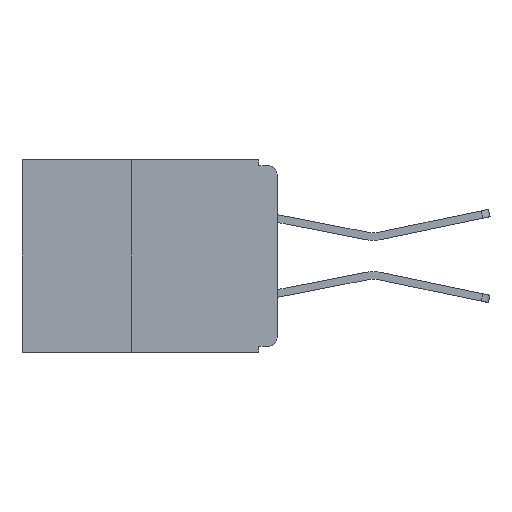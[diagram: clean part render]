
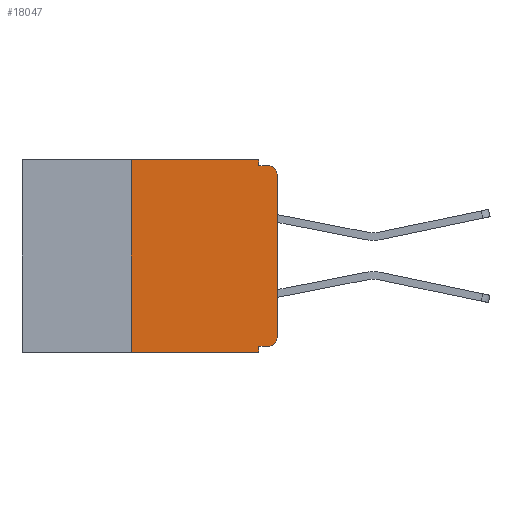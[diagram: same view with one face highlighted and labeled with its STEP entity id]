
A CAD part, left-side view. The second image highlights one B-rep face of the part: STEP entity #18047.
In plain terms, the highlighted planar face has unit normal (-1, 0, 0).
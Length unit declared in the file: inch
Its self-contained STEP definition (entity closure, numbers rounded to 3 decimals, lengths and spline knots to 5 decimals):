
#523 = VECTOR ( 'NONE', #11589, 39.37008 ) ;
#1470 = VERTEX_POINT ( 'NONE', #19646 ) ;
#1898 = VECTOR ( 'NONE', #27542, 39.37008 ) ;
#2054 = VECTOR ( 'NONE', #28961, 39.37008 ) ;
#2143 = VECTOR ( 'NONE', #12519, 39.37008 ) ;
#2217 = CIRCLE ( 'NONE', #30447, 0.015 ) ;
#2583 = ORIENTED_EDGE ( 'NONE', *, *, #22850, .F. ) ;
#2892 = VERTEX_POINT ( 'NONE', #30218 ) ;
#3573 = EDGE_CURVE ( 'NONE', #6749, #24442, #2217, .T. ) ;
#4048 = CARTESIAN_POINT ( 'NONE',  ( 0., 0.015, -0.01 ) ) ;
#4120 = DIRECTION ( 'NONE',  ( 0., 0., 1. ) ) ;
#5035 = VECTOR ( 'NONE', #14253, 39.37008 ) ;
#5167 = DIRECTION ( 'NONE',  ( 0., 0., -1. ) ) ;
#5255 = DIRECTION ( 'NONE',  ( -1., 0., 0. ) ) ;
#6128 = EDGE_CURVE ( 'NONE', #2892, #11223, #21045, .T. ) ;
#6496 = LINE ( 'NONE', #28523, #13029 ) ;
#6749 = VERTEX_POINT ( 'NONE', #17770 ) ;
#6940 = CARTESIAN_POINT ( 'NONE',  ( 0., 0.437, 0. ) ) ;
#6986 = CARTESIAN_POINT ( 'NONE',  ( 0., 0., -0.01 ) ) ;
#7570 = CARTESIAN_POINT ( 'NONE',  ( 0., 0.015, -0.32 ) ) ;
#8571 = LINE ( 'NONE', #6940, #2054 ) ;
#9008 = VERTEX_POINT ( 'NONE', #7570 ) ;
#9143 = CARTESIAN_POINT ( 'NONE',  ( 0., 0., -0.32 ) ) ;
#9176 = PLANE ( 'NONE',  #24827 ) ;
#9881 = CARTESIAN_POINT ( 'NONE',  ( 0., 0., -0.305 ) ) ;
#10434 = CARTESIAN_POINT ( 'NONE',  ( 0., 0.437, -0.33 ) ) ;
#10629 = CARTESIAN_POINT ( 'NONE',  ( 0., 0.25, -0.33 ) ) ;
#11039 = EDGE_CURVE ( 'NONE', #13516, #6749, #6496, .T. ) ;
#11223 = VERTEX_POINT ( 'NONE', #12266 ) ;
#11443 = VERTEX_POINT ( 'NONE', #30097 ) ;
#11589 = DIRECTION ( 'NONE',  ( 0., 1., 0. ) ) ;
#12009 = EDGE_CURVE ( 'NONE', #31217, #30993, #29386, .T. ) ;
#12266 = CARTESIAN_POINT ( 'NONE',  ( 0., 0.031, -0.33 ) ) ;
#12460 = CARTESIAN_POINT ( 'NONE',  ( 0., 0.031, -0.33 ) ) ;
#12519 = DIRECTION ( 'NONE',  ( 0., 0., -1. ) ) ;
#12658 = DIRECTION ( 'NONE',  ( 0., 0., 1. ) ) ;
#13029 = VECTOR ( 'NONE', #4120, 39.37008 ) ;
#13365 = LINE ( 'NONE', #10434, #1898 ) ;
#13516 = VERTEX_POINT ( 'NONE', #9881 ) ;
#14086 = CARTESIAN_POINT ( 'NONE',  ( 0., 0.437, 0. ) ) ;
#14253 = DIRECTION ( 'NONE',  ( 0., -1., 0. ) ) ;
#14514 = VECTOR ( 'NONE', #5167, 39.37008 ) ;
#14844 = EDGE_LOOP ( 'NONE', ( #20462, #28034, #19815, #2583, #19809, #22162, #22128, #17025, #21802, #21486 ) ) ;
#16553 = DIRECTION ( 'NONE',  ( 0., 0., -1. ) ) ;
#17025 = ORIENTED_EDGE ( 'NONE', *, *, #6128, .F. ) ;
#17576 = DIRECTION ( 'NONE',  ( 0., 0., -1. ) ) ;
#17614 = DIRECTION ( 'NONE',  ( -1., 0., 0. ) ) ;
#17640 = CARTESIAN_POINT ( 'NONE',  ( 0., 0.015, -0.025 ) ) ;
#17770 = CARTESIAN_POINT ( 'NONE',  ( 0., 0., -0.025 ) ) ;
#18047 = ADVANCED_FACE ( 'NONE', ( #25001 ), #9176, .F. ) ;
#18679 = EDGE_CURVE ( 'NONE', #9008, #2892, #20045, .T. ) ;
#19646 = CARTESIAN_POINT ( 'NONE',  ( 0., 0.031, -0.01 ) ) ;
#19735 = CARTESIAN_POINT ( 'NONE',  ( 0., 0.25, 0. ) ) ;
#19809 = ORIENTED_EDGE ( 'NONE', *, *, #29489, .F. ) ;
#19815 = ORIENTED_EDGE ( 'NONE', *, *, #31413, .F. ) ;
#19921 = CARTESIAN_POINT ( 'NONE',  ( 0., 0.015, -0.305 ) ) ;
#20033 = CARTESIAN_POINT ( 'NONE',  ( 0., 0.25, -0.33 ) ) ;
#20045 = LINE ( 'NONE', #9143, #523 ) ;
#20462 = ORIENTED_EDGE ( 'NONE', *, *, #11039, .T. ) ;
#20863 = EDGE_CURVE ( 'NONE', #31217, #11223, #13365, .T. ) ;
#20902 = LINE ( 'NONE', #27154, #2143 ) ;
#21045 = LINE ( 'NONE', #12460, #14514 ) ;
#21432 = EDGE_CURVE ( 'NONE', #9008, #13516, #22550, .T. ) ;
#21486 = ORIENTED_EDGE ( 'NONE', *, *, #21432, .T. ) ;
#21802 = ORIENTED_EDGE ( 'NONE', *, *, #18679, .F. ) ;
#22128 = ORIENTED_EDGE ( 'NONE', *, *, #20863, .T. ) ;
#22162 = ORIENTED_EDGE ( 'NONE', *, *, #12009, .F. ) ;
#22398 = DIRECTION ( 'NONE',  ( 0., 0., -1. ) ) ;
#22550 = CIRCLE ( 'NONE', #29594, 0.015 ) ;
#22850 = EDGE_CURVE ( 'NONE', #11443, #1470, #20902, .T. ) ;
#22918 = VECTOR ( 'NONE', #12658, 39.37008 ) ;
#24442 = VERTEX_POINT ( 'NONE', #4048 ) ;
#24827 = AXIS2_PLACEMENT_3D ( 'NONE', #14086, #31203, #16553 ) ;
#25001 = FACE_OUTER_BOUND ( 'NONE', #14844, .T. ) ;
#27154 = CARTESIAN_POINT ( 'NONE',  ( 0., 0.031, 0. ) ) ;
#27542 = DIRECTION ( 'NONE',  ( 0., -1., 0. ) ) ;
#28034 = ORIENTED_EDGE ( 'NONE', *, *, #3573, .T. ) ;
#28523 = CARTESIAN_POINT ( 'NONE',  ( 0., 0., 0. ) ) ;
#28961 = DIRECTION ( 'NONE',  ( 0., -1., 0. ) ) ;
#29386 = LINE ( 'NONE', #20033, #22918 ) ;
#29489 = EDGE_CURVE ( 'NONE', #30993, #11443, #8571, .T. ) ;
#29594 = AXIS2_PLACEMENT_3D ( 'NONE', #19921, #5255, #22398 ) ;
#30097 = CARTESIAN_POINT ( 'NONE',  ( 0., 0.031, 0. ) ) ;
#30218 = CARTESIAN_POINT ( 'NONE',  ( 0., 0.031, -0.32 ) ) ;
#30447 = AXIS2_PLACEMENT_3D ( 'NONE', #17640, #17614, #17576 ) ;
#30993 = VERTEX_POINT ( 'NONE', #19735 ) ;
#31060 = LINE ( 'NONE', #6986, #5035 ) ;
#31203 = DIRECTION ( 'NONE',  ( 1., 0., 0. ) ) ;
#31217 = VERTEX_POINT ( 'NONE', #10629 ) ;
#31413 = EDGE_CURVE ( 'NONE', #1470, #24442, #31060, .T. ) ;
